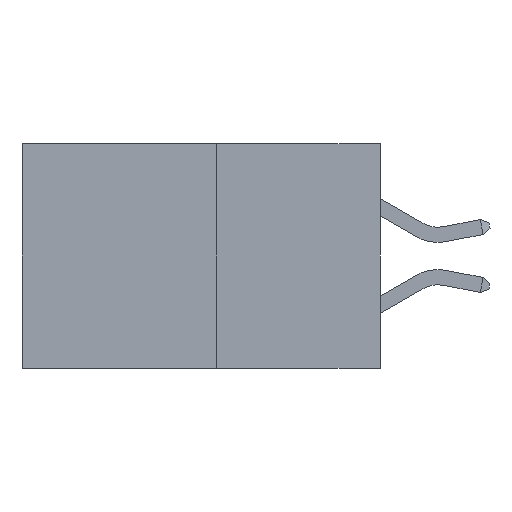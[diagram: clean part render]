
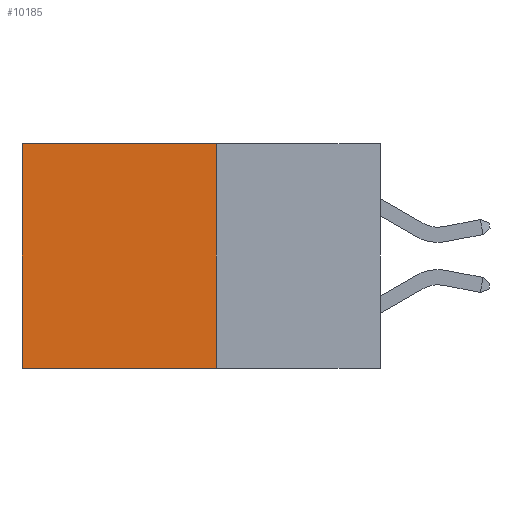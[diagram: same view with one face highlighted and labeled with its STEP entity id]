
A CAD part, left-side view. The second image highlights one B-rep face of the part: STEP entity #10185.
In plain terms, the highlighted planar face has unit normal (-1, 0, 0).
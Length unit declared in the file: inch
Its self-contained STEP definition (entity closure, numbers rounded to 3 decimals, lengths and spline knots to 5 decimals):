
#233 = FACE_OUTER_BOUND ( 'NONE', #9051, .T. ) ;
#380 = CARTESIAN_POINT ( 'NONE',  ( 0.277, 0.27, 0. ) ) ;
#662 = PLANE ( 'NONE',  #9431 ) ;
#1342 = CARTESIAN_POINT ( 'NONE',  ( 0.277, 0.59, -0.37 ) ) ;
#1664 = DIRECTION ( 'NONE',  ( 1., 0., 0. ) ) ;
#1704 = EDGE_CURVE ( 'NONE', #9448, #9547, #9176, .T. ) ;
#1773 = VERTEX_POINT ( 'NONE', #10008 ) ;
#1986 = ORIENTED_EDGE ( 'NONE', *, *, #5264, .T. ) ;
#2316 = ORIENTED_EDGE ( 'NONE', *, *, #1704, .T. ) ;
#2563 = CARTESIAN_POINT ( 'NONE',  ( 0.277, 0.27, -0.37 ) ) ;
#2700 = LINE ( 'NONE', #12351, #7720 ) ;
#5264 = EDGE_CURVE ( 'NONE', #9547, #6132, #2700, .T. ) ;
#5765 = VECTOR ( 'NONE', #6043, 39.37008 ) ;
#6043 = DIRECTION ( 'NONE',  ( 0., 1., 0. ) ) ;
#6132 = VERTEX_POINT ( 'NONE', #1342 ) ;
#6276 = VECTOR ( 'NONE', #10559, 39.37008 ) ;
#6512 = VECTOR ( 'NONE', #8344, 39.37008 ) ;
#7351 = ORIENTED_EDGE ( 'NONE', *, *, #11792, .F. ) ;
#7449 = EDGE_CURVE ( 'NONE', #9448, #1773, #11868, .T. ) ;
#7680 = CARTESIAN_POINT ( 'NONE',  ( 0.277, 0.27, -0.37 ) ) ;
#7720 = VECTOR ( 'NONE', #12115, 39.37008 ) ;
#8344 = DIRECTION ( 'NONE',  ( 0., 1., 0. ) ) ;
#8391 = CARTESIAN_POINT ( 'NONE',  ( 0.277, 0.27, 0. ) ) ;
#8689 = DIRECTION ( 'NONE',  ( 0., 0., -1. ) ) ;
#9051 = EDGE_LOOP ( 'NONE', ( #1986, #7351, #9995, #2316 ) ) ;
#9176 = LINE ( 'NONE', #8391, #6512 ) ;
#9431 = AXIS2_PLACEMENT_3D ( 'NONE', #7680, #1664, #8689 ) ;
#9448 = VERTEX_POINT ( 'NONE', #380 ) ;
#9547 = VERTEX_POINT ( 'NONE', #10651 ) ;
#9995 = ORIENTED_EDGE ( 'NONE', *, *, #7449, .F. ) ;
#10008 = CARTESIAN_POINT ( 'NONE',  ( 0.277, 0.27, -0.37 ) ) ;
#10185 = ADVANCED_FACE ( 'NONE', ( #233 ), #662, .F. ) ;
#10559 = DIRECTION ( 'NONE',  ( 0., 0., -1. ) ) ;
#10651 = CARTESIAN_POINT ( 'NONE',  ( 0.277, 0.59, 0. ) ) ;
#11039 = CARTESIAN_POINT ( 'NONE',  ( 0.277, 0.27, -0.37 ) ) ;
#11045 = LINE ( 'NONE', #11039, #5765 ) ;
#11792 = EDGE_CURVE ( 'NONE', #1773, #6132, #11045, .T. ) ;
#11868 = LINE ( 'NONE', #2563, #6276 ) ;
#12115 = DIRECTION ( 'NONE',  ( 0., 0., -1. ) ) ;
#12351 = CARTESIAN_POINT ( 'NONE',  ( 0.277, 0.59, -0.37 ) ) ;
